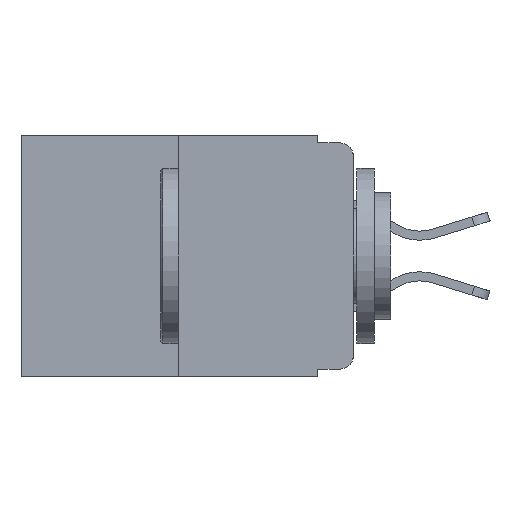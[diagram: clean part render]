
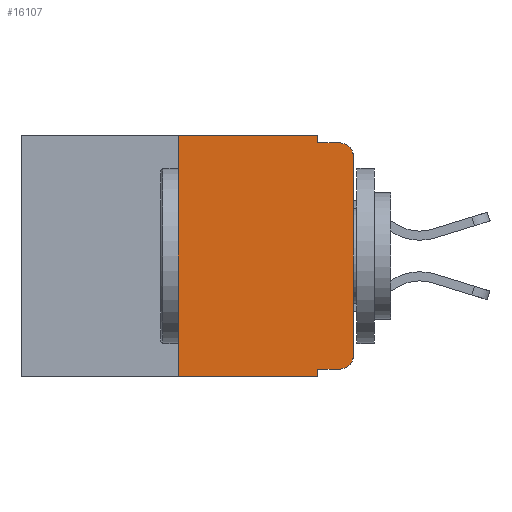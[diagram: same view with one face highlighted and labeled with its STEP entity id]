
A CAD part, left-side view. The second image highlights one B-rep face of the part: STEP entity #16107.
In plain terms, the highlighted planar face has unit normal (-1, 0, 0).
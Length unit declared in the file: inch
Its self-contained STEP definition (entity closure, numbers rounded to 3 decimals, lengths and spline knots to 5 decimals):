
#343 = LINE ( 'NONE', #21320, #19789 ) ;
#795 = ORIENTED_EDGE ( 'NONE', *, *, #17805, .F. ) ;
#931 = DIRECTION ( 'NONE',  ( 0., 0., -1. ) ) ;
#1631 = DIRECTION ( 'NONE',  ( 0., 0., -1. ) ) ;
#1999 = VECTOR ( 'NONE', #21985, 39.37008 ) ;
#2516 = CARTESIAN_POINT ( 'NONE',  ( 0., 0.02, -0.313 ) ) ;
#2624 = VERTEX_POINT ( 'NONE', #21274 ) ;
#2782 = FACE_OUTER_BOUND ( 'NONE', #7129, .T. ) ;
#3390 = DIRECTION ( 'NONE',  ( 0., 0., 1. ) ) ;
#3466 = VECTOR ( 'NONE', #23090, 39.37008 ) ;
#3677 = VERTEX_POINT ( 'NONE', #13191 ) ;
#3794 = VERTEX_POINT ( 'NONE', #11733 ) ;
#3902 = PLANE ( 'NONE',  #22777 ) ;
#4141 = ORIENTED_EDGE ( 'NONE', *, *, #11047, .T. ) ;
#4221 = CIRCLE ( 'NONE', #21169, 0.02 ) ;
#4288 = VECTOR ( 'NONE', #1631, 39.37008 ) ;
#4402 = DIRECTION ( 'NONE',  ( -1., 0., 0. ) ) ;
#5001 = CARTESIAN_POINT ( 'NONE',  ( 0., 0., -0.313 ) ) ;
#5069 = VERTEX_POINT ( 'NONE', #12738 ) ;
#5540 = DIRECTION ( 'NONE',  ( 0., -1., 0. ) ) ;
#5814 = ORIENTED_EDGE ( 'NONE', *, *, #16541, .F. ) ;
#6665 = ORIENTED_EDGE ( 'NONE', *, *, #13790, .T. ) ;
#6729 = LINE ( 'NONE', #22551, #4288 ) ;
#7129 = EDGE_LOOP ( 'NONE', ( #6665, #4141, #20032, #5814, #19485, #795, #17969, #9208, #11339, #20473 ) ) ;
#7233 = CARTESIAN_POINT ( 'NONE',  ( 0., 0.25, 0. ) ) ;
#7274 = VECTOR ( 'NONE', #10702, 39.37008 ) ;
#7568 = DIRECTION ( 'NONE',  ( 0., 0., -1. ) ) ;
#7941 = VECTOR ( 'NONE', #3390, 39.37008 ) ;
#8269 = CIRCLE ( 'NONE', #22359, 0.02 ) ;
#8327 = CARTESIAN_POINT ( 'NONE',  ( 0., 0.051, -0.333 ) ) ;
#8655 = DIRECTION ( 'NONE',  ( 0., -1., 0. ) ) ;
#8727 = CARTESIAN_POINT ( 'NONE',  ( 0., 0.051, 0. ) ) ;
#8831 = DIRECTION ( 'NONE',  ( -1., 0., 0. ) ) ;
#8910 = CARTESIAN_POINT ( 'NONE',  ( 0., 0.473, -0.343 ) ) ;
#9039 = VERTEX_POINT ( 'NONE', #5001 ) ;
#9208 = ORIENTED_EDGE ( 'NONE', *, *, #24136, .F. ) ;
#9884 = CARTESIAN_POINT ( 'NONE',  ( 0., 0.051, 0. ) ) ;
#10386 = LINE ( 'NONE', #20275, #7274 ) ;
#10702 = DIRECTION ( 'NONE',  ( 0., -1., 0. ) ) ;
#10752 = CARTESIAN_POINT ( 'NONE',  ( 0., 0.02, -0.03 ) ) ;
#11047 = EDGE_CURVE ( 'NONE', #3794, #2624, #8269, .T. ) ;
#11339 = ORIENTED_EDGE ( 'NONE', *, *, #15377, .T. ) ;
#11400 = VECTOR ( 'NONE', #14177, 39.37008 ) ;
#11733 = CARTESIAN_POINT ( 'NONE',  ( 0., 0., -0.03 ) ) ;
#12171 = EDGE_CURVE ( 'NONE', #5069, #2624, #10386, .T. ) ;
#12517 = VERTEX_POINT ( 'NONE', #8727 ) ;
#12738 = CARTESIAN_POINT ( 'NONE',  ( 0., 0.051, -0.01 ) ) ;
#13191 = CARTESIAN_POINT ( 'NONE',  ( 0., 0.051, -0.343 ) ) ;
#13790 = EDGE_CURVE ( 'NONE', #9039, #3794, #16777, .T. ) ;
#14177 = DIRECTION ( 'NONE',  ( 0., 0., -1. ) ) ;
#15377 = EDGE_CURVE ( 'NONE', #24431, #20058, #343, .T. ) ;
#15759 = LINE ( 'NONE', #8910, #17634 ) ;
#16107 = ADVANCED_FACE ( 'NONE', ( #2782 ), #3902, .F. ) ;
#16113 = DIRECTION ( 'NONE',  ( 0., 0., -1. ) ) ;
#16541 = EDGE_CURVE ( 'NONE', #12517, #5069, #6729, .T. ) ;
#16777 = LINE ( 'NONE', #20008, #1999 ) ;
#17329 = LINE ( 'NONE', #23429, #3466 ) ;
#17634 = VECTOR ( 'NONE', #8655, 39.37008 ) ;
#17805 = EDGE_CURVE ( 'NONE', #21776, #17831, #25211, .T. ) ;
#17831 = VERTEX_POINT ( 'NONE', #7233 ) ;
#17876 = LINE ( 'NONE', #9884, #11400 ) ;
#17969 = ORIENTED_EDGE ( 'NONE', *, *, #23209, .T. ) ;
#18767 = EDGE_CURVE ( 'NONE', #20058, #9039, #4221, .T. ) ;
#19485 = ORIENTED_EDGE ( 'NONE', *, *, #22806, .F. ) ;
#19662 = DIRECTION ( 'NONE',  ( 1., 0., 0. ) ) ;
#19789 = VECTOR ( 'NONE', #5540, 39.37008 ) ;
#20008 = CARTESIAN_POINT ( 'NONE',  ( 0., 0., 0. ) ) ;
#20032 = ORIENTED_EDGE ( 'NONE', *, *, #12171, .F. ) ;
#20058 = VERTEX_POINT ( 'NONE', #22084 ) ;
#20275 = CARTESIAN_POINT ( 'NONE',  ( 0., 0.051, -0.01 ) ) ;
#20473 = ORIENTED_EDGE ( 'NONE', *, *, #18767, .T. ) ;
#21169 = AXIS2_PLACEMENT_3D ( 'NONE', #2516, #4402, #16113 ) ;
#21274 = CARTESIAN_POINT ( 'NONE',  ( 0., 0.02, -0.01 ) ) ;
#21320 = CARTESIAN_POINT ( 'NONE',  ( 0., 0.051, -0.333 ) ) ;
#21776 = VERTEX_POINT ( 'NONE', #23396 ) ;
#21985 = DIRECTION ( 'NONE',  ( 0., 0., 1. ) ) ;
#22084 = CARTESIAN_POINT ( 'NONE',  ( 0., 0.02, -0.333 ) ) ;
#22359 = AXIS2_PLACEMENT_3D ( 'NONE', #10752, #8831, #931 ) ;
#22551 = CARTESIAN_POINT ( 'NONE',  ( 0., 0.051, 0. ) ) ;
#22777 = AXIS2_PLACEMENT_3D ( 'NONE', #23439, #19662, #7568 ) ;
#22806 = EDGE_CURVE ( 'NONE', #17831, #12517, #17329, .T. ) ;
#23090 = DIRECTION ( 'NONE',  ( 0., -1., 0. ) ) ;
#23103 = CARTESIAN_POINT ( 'NONE',  ( 0., 0.25, 0. ) ) ;
#23209 = EDGE_CURVE ( 'NONE', #21776, #3677, #15759, .T. ) ;
#23396 = CARTESIAN_POINT ( 'NONE',  ( 0., 0.25, -0.343 ) ) ;
#23429 = CARTESIAN_POINT ( 'NONE',  ( 0., 0.473, 0. ) ) ;
#23439 = CARTESIAN_POINT ( 'NONE',  ( 0., 0.473, 0. ) ) ;
#24136 = EDGE_CURVE ( 'NONE', #24431, #3677, #17876, .T. ) ;
#24431 = VERTEX_POINT ( 'NONE', #8327 ) ;
#25211 = LINE ( 'NONE', #23103, #7941 ) ;
